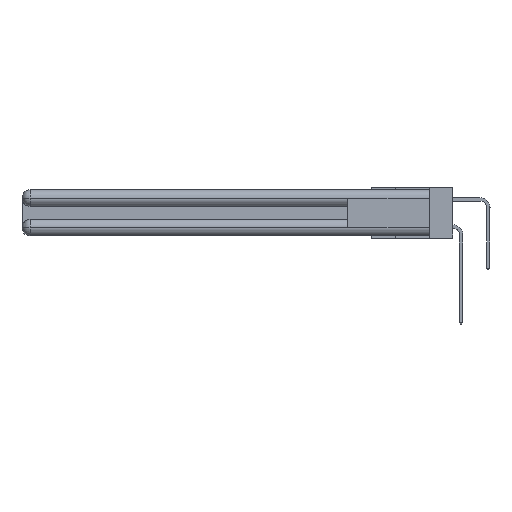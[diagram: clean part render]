
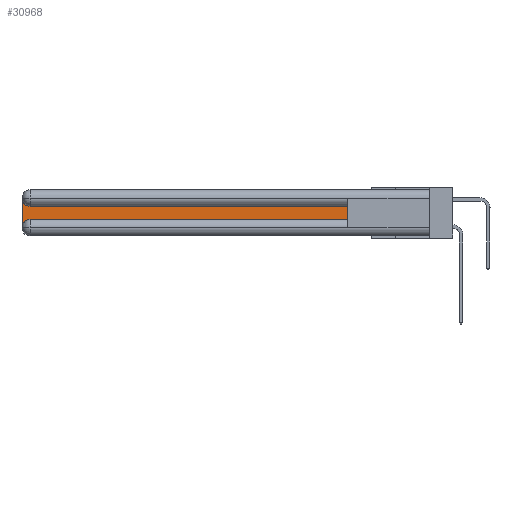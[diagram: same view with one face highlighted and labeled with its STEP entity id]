
A CAD part, left-side view. The second image highlights one B-rep face of the part: STEP entity #30968.
In plain terms, the highlighted planar face has unit normal (-1, 0, 0).
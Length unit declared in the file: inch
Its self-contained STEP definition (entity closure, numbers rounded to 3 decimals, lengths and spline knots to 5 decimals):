
#273 = DIRECTION ( 'NONE',  ( 0., 0., -1. ) ) ;
#361 = ORIENTED_EDGE ( 'NONE', *, *, #21862, .T. ) ;
#715 = VERTEX_POINT ( 'NONE', #3681 ) ;
#1430 = CARTESIAN_POINT ( 'NONE',  ( 0.075, 2.94, -0.0625 ) ) ;
#2014 = EDGE_CURVE ( 'NONE', #19449, #30488, #11056, .T. ) ;
#2197 = DIRECTION ( 'NONE',  ( 0., 0., -1. ) ) ;
#3681 = CARTESIAN_POINT ( 'NONE',  ( 0.075, 2.94, -0.2175 ) ) ;
#3836 = VECTOR ( 'NONE', #5480, 39.37008 ) ;
#4366 = CARTESIAN_POINT ( 'NONE',  ( 0.075, 0.6, -0.1225 ) ) ;
#5002 = VECTOR ( 'NONE', #9429, 39.37008 ) ;
#5480 = DIRECTION ( 'NONE',  ( 0., -1., 0. ) ) ;
#6445 = CARTESIAN_POINT ( 'NONE',  ( 0.075, 0.6, -0.2175 ) ) ;
#7150 = CARTESIAN_POINT ( 'NONE',  ( 0.075, 3., -0.2175 ) ) ;
#7869 = ORIENTED_EDGE ( 'NONE', *, *, #23260, .T. ) ;
#8844 = LINE ( 'NONE', #7150, #10030 ) ;
#8992 = DIRECTION ( 'NONE',  ( 0., 0., 1. ) ) ;
#9429 = DIRECTION ( 'NONE',  ( 0., 1., 0. ) ) ;
#10030 = VECTOR ( 'NONE', #2197, 39.37008 ) ;
#10832 = VECTOR ( 'NONE', #8992, 39.37008 ) ;
#11056 = CIRCLE ( 'NONE', #16573, 0.06 ) ;
#11322 = DIRECTION ( 'NONE',  ( 1., 0., 0. ) ) ;
#11971 = VERTEX_POINT ( 'NONE', #15316 ) ;
#13609 = CARTESIAN_POINT ( 'NONE',  ( 0.075, 2.94, -0.1225 ) ) ;
#14136 = DIRECTION ( 'NONE',  ( 0., 0., -1. ) ) ;
#14542 = CIRCLE ( 'NONE', #15234, 0.06 ) ;
#15089 = ORIENTED_EDGE ( 'NONE', *, *, #24376, .T. ) ;
#15234 = AXIS2_PLACEMENT_3D ( 'NONE', #21109, #11322, #21001 ) ;
#15316 = CARTESIAN_POINT ( 'NONE',  ( 0.075, 0.6, -0.1225 ) ) ;
#16573 = AXIS2_PLACEMENT_3D ( 'NONE', #1430, #21874, #14136 ) ;
#17593 = EDGE_CURVE ( 'NONE', #29371, #11971, #27762, .T. ) ;
#18037 = LINE ( 'NONE', #23184, #3836 ) ;
#19449 = VERTEX_POINT ( 'NONE', #13609 ) ;
#21001 = DIRECTION ( 'NONE',  ( 0., 0., -1. ) ) ;
#21109 = CARTESIAN_POINT ( 'NONE',  ( 0.075, 2.94, -0.2775 ) ) ;
#21862 = EDGE_CURVE ( 'NONE', #32522, #715, #14542, .T. ) ;
#21874 = DIRECTION ( 'NONE',  ( 1., 0., 0. ) ) ;
#22092 = CARTESIAN_POINT ( 'NONE',  ( 0.075, 3., -0.0625 ) ) ;
#22819 = PLANE ( 'NONE',  #27138 ) ;
#23184 = CARTESIAN_POINT ( 'NONE',  ( 0.075, 0.6, -0.2175 ) ) ;
#23260 = EDGE_CURVE ( 'NONE', #11971, #19449, #32186, .T. ) ;
#23698 = FACE_OUTER_BOUND ( 'NONE', #25792, .T. ) ;
#24376 = EDGE_CURVE ( 'NONE', #30488, #32522, #8844, .T. ) ;
#25234 = ORIENTED_EDGE ( 'NONE', *, *, #17593, .T. ) ;
#25344 = CARTESIAN_POINT ( 'NONE',  ( 0.075, 3., -0.1225 ) ) ;
#25792 = EDGE_LOOP ( 'NONE', ( #7869, #30843, #15089, #361, #29289, #25234 ) ) ;
#25831 = EDGE_CURVE ( 'NONE', #715, #29371, #18037, .T. ) ;
#27138 = AXIS2_PLACEMENT_3D ( 'NONE', #25344, #32559, #273 ) ;
#27762 = LINE ( 'NONE', #6445, #10832 ) ;
#29037 = CARTESIAN_POINT ( 'NONE',  ( 0.075, 3., -0.2775 ) ) ;
#29289 = ORIENTED_EDGE ( 'NONE', *, *, #25831, .T. ) ;
#29371 = VERTEX_POINT ( 'NONE', #30385 ) ;
#30385 = CARTESIAN_POINT ( 'NONE',  ( 0.075, 0.6, -0.2175 ) ) ;
#30488 = VERTEX_POINT ( 'NONE', #22092 ) ;
#30843 = ORIENTED_EDGE ( 'NONE', *, *, #2014, .T. ) ;
#30968 = ADVANCED_FACE ( 'NONE', ( #23698 ), #22819, .F. ) ;
#32186 = LINE ( 'NONE', #4366, #5002 ) ;
#32522 = VERTEX_POINT ( 'NONE', #29037 ) ;
#32559 = DIRECTION ( 'NONE',  ( 1., 0., 0. ) ) ;
